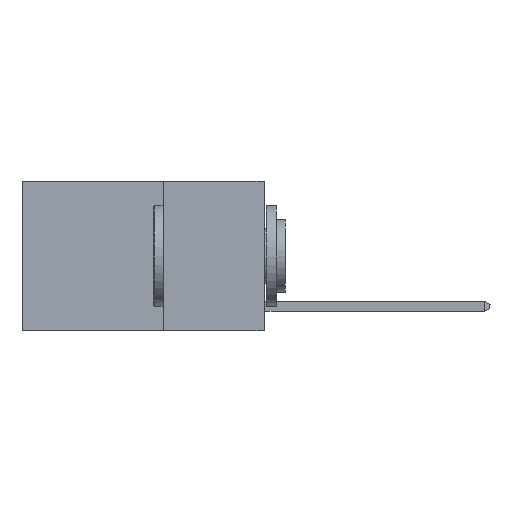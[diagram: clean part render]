
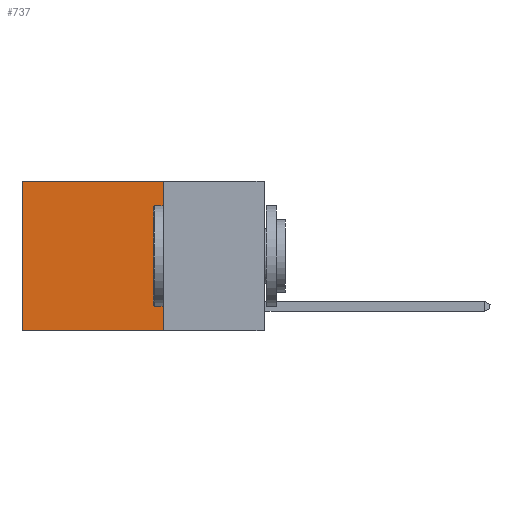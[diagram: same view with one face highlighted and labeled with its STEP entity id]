
A CAD part, left-side view. The second image highlights one B-rep face of the part: STEP entity #737.
In plain terms, the highlighted planar face has unit normal (-1, 0, 0).
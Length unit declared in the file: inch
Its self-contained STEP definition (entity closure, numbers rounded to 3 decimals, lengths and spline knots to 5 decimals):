
#490 = CARTESIAN_POINT ( 'NONE',  ( 0.2625, 0.6, 0. ) ) ;
#545 = VERTEX_POINT ( 'NONE', #16922 ) ;
#737 = ADVANCED_FACE ( 'NONE', ( #20245 ), #24301, .F. ) ;
#854 = CARTESIAN_POINT ( 'NONE',  ( 0.2625, 0.25, 0. ) ) ;
#1320 = EDGE_LOOP ( 'NONE', ( #21274, #6234, #20162, #16982 ) ) ;
#1634 = CARTESIAN_POINT ( 'NONE',  ( 0.2625, 0.25, 0. ) ) ;
#1762 = LINE ( 'NONE', #21421, #11100 ) ;
#2301 = EDGE_CURVE ( 'NONE', #4013, #545, #4870, .T. ) ;
#4013 = VERTEX_POINT ( 'NONE', #1634 ) ;
#4540 = CARTESIAN_POINT ( 'NONE',  ( 0.2625, 0.25, -0.37 ) ) ;
#4870 = LINE ( 'NONE', #9224, #24282 ) ;
#6104 = EDGE_CURVE ( 'NONE', #16920, #15238, #1762, .T. ) ;
#6234 = ORIENTED_EDGE ( 'NONE', *, *, #20530, .F. ) ;
#8595 = LINE ( 'NONE', #4540, #23636 ) ;
#9224 = CARTESIAN_POINT ( 'NONE',  ( 0.2625, 0.25, 0. ) ) ;
#11100 = VECTOR ( 'NONE', #13880, 39.37008 ) ;
#11174 = LINE ( 'NONE', #15405, #16232 ) ;
#11593 = DIRECTION ( 'NONE',  ( 0., 1., 0. ) ) ;
#13880 = DIRECTION ( 'NONE',  ( 0., 0., -1. ) ) ;
#15238 = VERTEX_POINT ( 'NONE', #18030 ) ;
#15405 = CARTESIAN_POINT ( 'NONE',  ( 0.2625, 0.25, 0. ) ) ;
#15676 = EDGE_CURVE ( 'NONE', #4013, #16920, #11174, .T. ) ;
#15818 = DIRECTION ( 'NONE',  ( 0., 1., 0. ) ) ;
#16232 = VECTOR ( 'NONE', #11593, 39.37008 ) ;
#16920 = VERTEX_POINT ( 'NONE', #490 ) ;
#16922 = CARTESIAN_POINT ( 'NONE',  ( 0.2625, 0.25, -0.37 ) ) ;
#16982 = ORIENTED_EDGE ( 'NONE', *, *, #15676, .T. ) ;
#17576 = AXIS2_PLACEMENT_3D ( 'NONE', #854, #23885, #23838 ) ;
#18030 = CARTESIAN_POINT ( 'NONE',  ( 0.2625, 0.6, -0.37 ) ) ;
#18837 = DIRECTION ( 'NONE',  ( 0., 0., -1. ) ) ;
#20162 = ORIENTED_EDGE ( 'NONE', *, *, #2301, .F. ) ;
#20245 = FACE_OUTER_BOUND ( 'NONE', #1320, .T. ) ;
#20530 = EDGE_CURVE ( 'NONE', #545, #15238, #8595, .T. ) ;
#21274 = ORIENTED_EDGE ( 'NONE', *, *, #6104, .T. ) ;
#21421 = CARTESIAN_POINT ( 'NONE',  ( 0.2625, 0.6, 0. ) ) ;
#23636 = VECTOR ( 'NONE', #15818, 39.37008 ) ;
#23838 = DIRECTION ( 'NONE',  ( 0., 0., -1. ) ) ;
#23885 = DIRECTION ( 'NONE',  ( 1., 0., 0. ) ) ;
#24282 = VECTOR ( 'NONE', #18837, 39.37008 ) ;
#24301 = PLANE ( 'NONE',  #17576 ) ;
